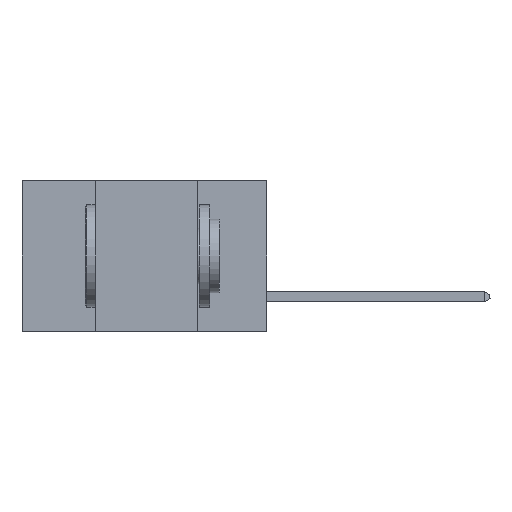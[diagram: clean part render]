
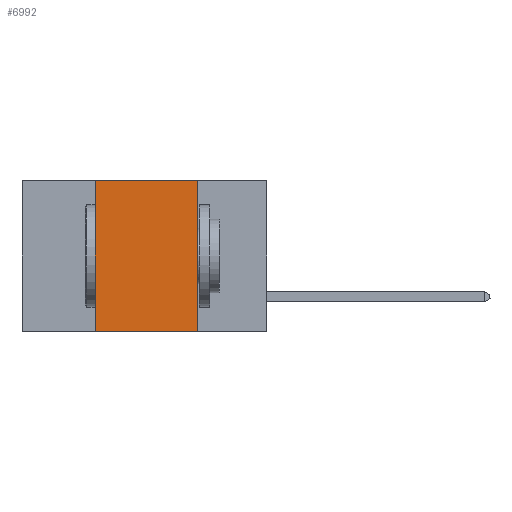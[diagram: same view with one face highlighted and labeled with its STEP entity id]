
A CAD part, left-side view. The second image highlights one B-rep face of the part: STEP entity #6992.
In plain terms, the highlighted planar face has unit normal (-1, 0, 0).
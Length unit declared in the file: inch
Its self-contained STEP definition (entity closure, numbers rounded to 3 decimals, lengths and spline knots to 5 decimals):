
#538 = CARTESIAN_POINT ( 'NONE',  ( 0., 0.17, 0. ) ) ;
#621 = EDGE_CURVE ( 'NONE', #3360, #7997, #2552, .T. ) ;
#2063 = VERTEX_POINT ( 'NONE', #5835 ) ;
#2331 = CARTESIAN_POINT ( 'NONE',  ( 0., 0.17, 0. ) ) ;
#2384 = DIRECTION ( 'NONE',  ( 0., 0., -1. ) ) ;
#2552 = LINE ( 'NONE', #7636, #7087 ) ;
#2994 = VECTOR ( 'NONE', #9122, 39.37008 ) ;
#3360 = VERTEX_POINT ( 'NONE', #4308 ) ;
#3511 = EDGE_CURVE ( 'NONE', #10040, #2063, #3575, .T. ) ;
#3575 = LINE ( 'NONE', #5297, #7985 ) ;
#4308 = CARTESIAN_POINT ( 'NONE',  ( 0., 0.42, 0. ) ) ;
#4367 = DIRECTION ( 'NONE',  ( 0., -1., 0. ) ) ;
#4448 = LINE ( 'NONE', #2331, #2994 ) ;
#4483 = DIRECTION ( 'NONE',  ( 0., -1., 0. ) ) ;
#4990 = EDGE_CURVE ( 'NONE', #7997, #2063, #4448, .T. ) ;
#5297 = CARTESIAN_POINT ( 'NONE',  ( 0., 0.6, -0.37 ) ) ;
#5465 = FACE_OUTER_BOUND ( 'NONE', #9492, .T. ) ;
#5835 = CARTESIAN_POINT ( 'NONE',  ( 0., 0.17, -0.37 ) ) ;
#5982 = LINE ( 'NONE', #7711, #6363 ) ;
#6363 = VECTOR ( 'NONE', #7812, 39.37008 ) ;
#6404 = AXIS2_PLACEMENT_3D ( 'NONE', #6511, #10763, #2384 ) ;
#6511 = CARTESIAN_POINT ( 'NONE',  ( 0., 0.6, 0. ) ) ;
#6588 = PLANE ( 'NONE',  #6404 ) ;
#6992 = ADVANCED_FACE ( 'NONE', ( #5465 ), #6588, .F. ) ;
#6993 = ORIENTED_EDGE ( 'NONE', *, *, #621, .F. ) ;
#7087 = VECTOR ( 'NONE', #4367, 39.37008 ) ;
#7229 = EDGE_CURVE ( 'NONE', #10040, #3360, #5982, .T. ) ;
#7401 = CARTESIAN_POINT ( 'NONE',  ( 0., 0.42, -0.37 ) ) ;
#7636 = CARTESIAN_POINT ( 'NONE',  ( 0., 0.6, 0. ) ) ;
#7711 = CARTESIAN_POINT ( 'NONE',  ( 0., 0.42, 0. ) ) ;
#7812 = DIRECTION ( 'NONE',  ( 0., 0., 1. ) ) ;
#7985 = VECTOR ( 'NONE', #4483, 39.37008 ) ;
#7997 = VERTEX_POINT ( 'NONE', #538 ) ;
#8331 = ORIENTED_EDGE ( 'NONE', *, *, #3511, .T. ) ;
#8669 = ORIENTED_EDGE ( 'NONE', *, *, #4990, .F. ) ;
#9092 = ORIENTED_EDGE ( 'NONE', *, *, #7229, .F. ) ;
#9122 = DIRECTION ( 'NONE',  ( 0., 0., -1. ) ) ;
#9492 = EDGE_LOOP ( 'NONE', ( #8669, #6993, #9092, #8331 ) ) ;
#10040 = VERTEX_POINT ( 'NONE', #7401 ) ;
#10763 = DIRECTION ( 'NONE',  ( 1., 0., 0. ) ) ;
